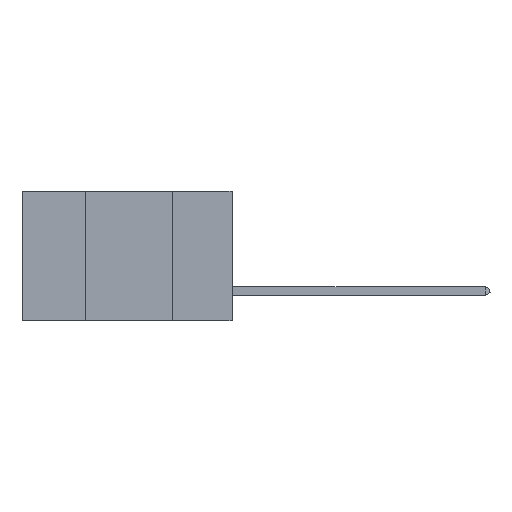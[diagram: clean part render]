
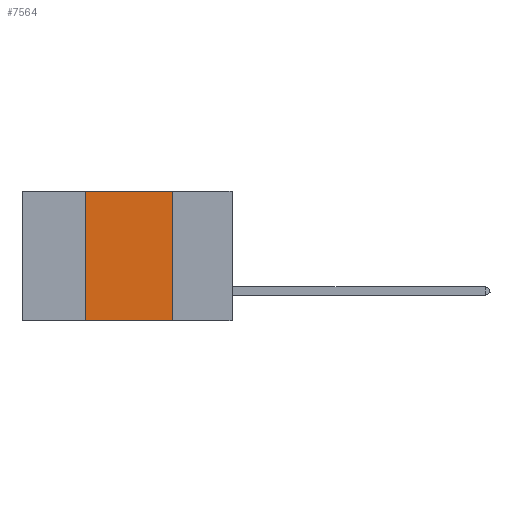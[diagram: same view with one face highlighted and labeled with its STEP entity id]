
A CAD part, left-side view. The second image highlights one B-rep face of the part: STEP entity #7564.
In plain terms, the highlighted planar face has unit normal (-1, 0, 0).
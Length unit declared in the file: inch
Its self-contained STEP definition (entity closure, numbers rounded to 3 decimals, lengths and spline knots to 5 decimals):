
#601 = LINE ( 'NONE', #11290, #11319 ) ;
#777 = VECTOR ( 'NONE', #18371, 39.37008 ) ;
#1812 = ORIENTED_EDGE ( 'NONE', *, *, #17700, .T. ) ;
#3395 = ORIENTED_EDGE ( 'NONE', *, *, #6892, .F. ) ;
#3594 = VERTEX_POINT ( 'NONE', #11026 ) ;
#3937 = DIRECTION ( 'NONE',  ( 0., 0., 1. ) ) ;
#3967 = DIRECTION ( 'NONE',  ( 0., -1., 0. ) ) ;
#4599 = VERTEX_POINT ( 'NONE', #10614 ) ;
#4754 = ORIENTED_EDGE ( 'NONE', *, *, #15978, .F. ) ;
#5272 = CARTESIAN_POINT ( 'NONE',  ( 0., 0.6, -0.37 ) ) ;
#6892 = EDGE_CURVE ( 'NONE', #4599, #18107, #7754, .T. ) ;
#7564 = ADVANCED_FACE ( 'NONE', ( #10871 ), #17687, .F. ) ;
#7602 = EDGE_CURVE ( 'NONE', #18107, #11228, #601, .T. ) ;
#7754 = LINE ( 'NONE', #10769, #12258 ) ;
#8564 = CARTESIAN_POINT ( 'NONE',  ( 0., 0.17, 0. ) ) ;
#10614 = CARTESIAN_POINT ( 'NONE',  ( 0., 0.42, -0.37 ) ) ;
#10769 = CARTESIAN_POINT ( 'NONE',  ( 0., 0.42, 0. ) ) ;
#10871 = FACE_OUTER_BOUND ( 'NONE', #12598, .T. ) ;
#11026 = CARTESIAN_POINT ( 'NONE',  ( 0., 0.17, -0.37 ) ) ;
#11228 = VERTEX_POINT ( 'NONE', #13841 ) ;
#11290 = CARTESIAN_POINT ( 'NONE',  ( 0., 0.6, 0. ) ) ;
#11319 = VECTOR ( 'NONE', #3967, 39.37008 ) ;
#12258 = VECTOR ( 'NONE', #3937, 39.37008 ) ;
#12441 = DIRECTION ( 'NONE',  ( 0., 0., -1. ) ) ;
#12598 = EDGE_LOOP ( 'NONE', ( #4754, #12699, #3395, #1812 ) ) ;
#12699 = ORIENTED_EDGE ( 'NONE', *, *, #7602, .F. ) ;
#13841 = CARTESIAN_POINT ( 'NONE',  ( 0., 0.17, 0. ) ) ;
#14552 = VECTOR ( 'NONE', #16678, 39.37008 ) ;
#15180 = CARTESIAN_POINT ( 'NONE',  ( 0., 0.6, 0. ) ) ;
#15978 = EDGE_CURVE ( 'NONE', #11228, #3594, #18445, .T. ) ;
#16678 = DIRECTION ( 'NONE',  ( 0., -1., 0. ) ) ;
#17404 = AXIS2_PLACEMENT_3D ( 'NONE', #15180, #18144, #12441 ) ;
#17588 = CARTESIAN_POINT ( 'NONE',  ( 0., 0.42, 0. ) ) ;
#17687 = PLANE ( 'NONE',  #17404 ) ;
#17700 = EDGE_CURVE ( 'NONE', #4599, #3594, #18373, .T. ) ;
#18107 = VERTEX_POINT ( 'NONE', #17588 ) ;
#18144 = DIRECTION ( 'NONE',  ( 1., 0., 0. ) ) ;
#18371 = DIRECTION ( 'NONE',  ( 0., 0., -1. ) ) ;
#18373 = LINE ( 'NONE', #5272, #14552 ) ;
#18445 = LINE ( 'NONE', #8564, #777 ) ;
